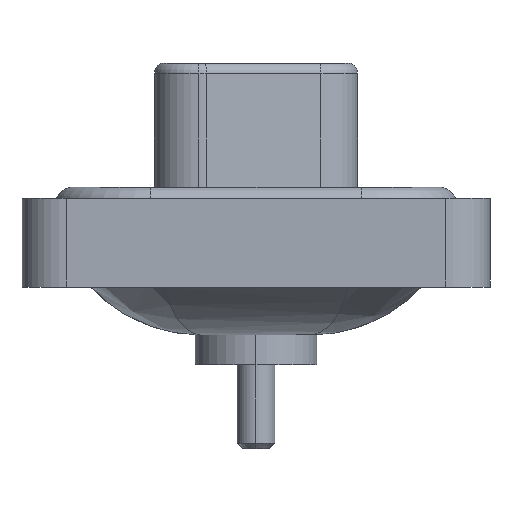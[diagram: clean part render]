
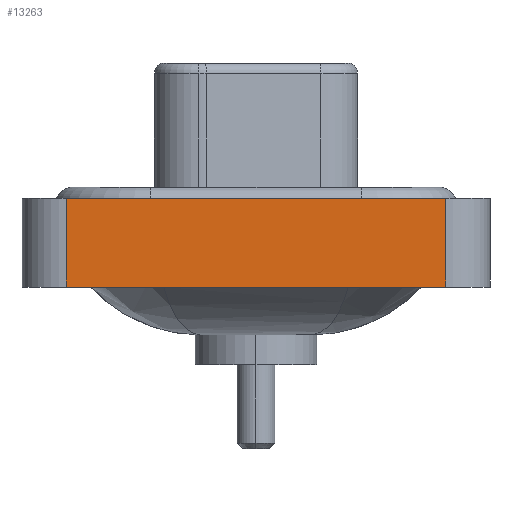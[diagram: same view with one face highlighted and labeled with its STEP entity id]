
A CAD part, left-side view. The second image highlights one B-rep face of the part: STEP entity #13263.
In plain terms, the highlighted planar face has unit normal (-1, 0, 0).
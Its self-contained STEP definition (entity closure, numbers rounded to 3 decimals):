
#184 = ORIENTED_EDGE ( 'NONE', *, *, #5906, .T. ) ;
#858 = CARTESIAN_POINT ( 'NONE',  ( -7.25, 8.55, -3.6 ) ) ;
#1254 = LINE ( 'NONE', #5194, #11189 ) ;
#1940 = DIRECTION ( 'NONE',  ( 0., 0., 1. ) ) ;
#1997 = EDGE_CURVE ( 'NONE', #10917, #3272, #11434, .T. ) ;
#2031 = DIRECTION ( 'NONE',  ( 0., 0., 1. ) ) ;
#2045 = EDGE_CURVE ( 'NONE', #10917, #3140, #8894, .T. ) ;
#2665 = AXIS2_PLACEMENT_3D ( 'NONE', #4697, #8805, #2031 ) ;
#3140 = VERTEX_POINT ( 'NONE', #13150 ) ;
#3147 = FACE_OUTER_BOUND ( 'NONE', #9461, .T. ) ;
#3182 = ORIENTED_EDGE ( 'NONE', *, *, #2045, .F. ) ;
#3272 = VERTEX_POINT ( 'NONE', #9417 ) ;
#3417 = ORIENTED_EDGE ( 'NONE', *, *, #1997, .T. ) ;
#4527 = EDGE_CURVE ( 'NONE', #3140, #14452, #14997, .T. ) ;
#4697 = CARTESIAN_POINT ( 'NONE',  ( -7.25, -8.55, -3.6 ) ) ;
#5194 = CARTESIAN_POINT ( 'NONE',  ( -7.25, -8.55, -3.6 ) ) ;
#5816 = CARTESIAN_POINT ( 'NONE',  ( -7.25, 8.55, -3.6 ) ) ;
#5906 = EDGE_CURVE ( 'NONE', #3272, #14452, #1254, .T. ) ;
#6356 = DIRECTION ( 'NONE',  ( 0., 0., 1. ) ) ;
#7535 = CARTESIAN_POINT ( 'NONE',  ( -7.25, -8.55, -3.6 ) ) ;
#8805 = DIRECTION ( 'NONE',  ( -1., 0., 0. ) ) ;
#8894 = LINE ( 'NONE', #5816, #12185 ) ;
#9417 = CARTESIAN_POINT ( 'NONE',  ( -7.25, -8.55, -3.6 ) ) ;
#9461 = EDGE_LOOP ( 'NONE', ( #184, #14170, #3182, #3417 ) ) ;
#10917 = VERTEX_POINT ( 'NONE', #858 ) ;
#11189 = VECTOR ( 'NONE', #6356, 1000. ) ;
#11434 = LINE ( 'NONE', #7535, #11894 ) ;
#11894 = VECTOR ( 'NONE', #16964, 1000. ) ;
#12185 = VECTOR ( 'NONE', #1940, 1000. ) ;
#12280 = DIRECTION ( 'NONE',  ( 0., -1., 0. ) ) ;
#13150 = CARTESIAN_POINT ( 'NONE',  ( -7.25, 8.55, 0.4 ) ) ;
#13263 = ADVANCED_FACE ( 'NONE', ( #3147 ), #14426, .T. ) ;
#14170 = ORIENTED_EDGE ( 'NONE', *, *, #4527, .F. ) ;
#14426 = PLANE ( 'NONE',  #2665 ) ;
#14452 = VERTEX_POINT ( 'NONE', #15281 ) ;
#14818 = CARTESIAN_POINT ( 'NONE',  ( -7.25, -8.55, 0.4 ) ) ;
#14997 = LINE ( 'NONE', #14818, #15198 ) ;
#15198 = VECTOR ( 'NONE', #12280, 1000. ) ;
#15281 = CARTESIAN_POINT ( 'NONE',  ( -7.25, -8.55, 0.4 ) ) ;
#16964 = DIRECTION ( 'NONE',  ( 0., -1., 0. ) ) ;
